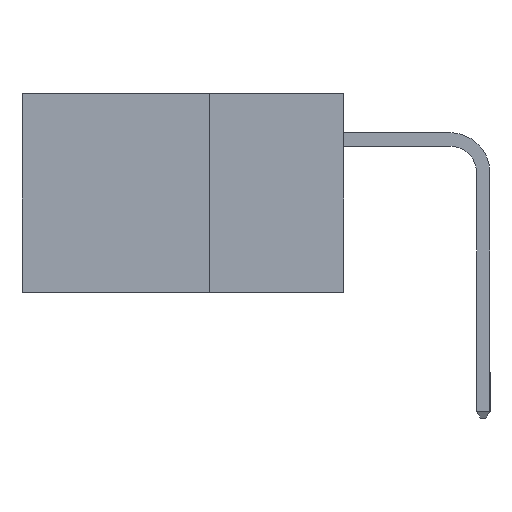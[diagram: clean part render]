
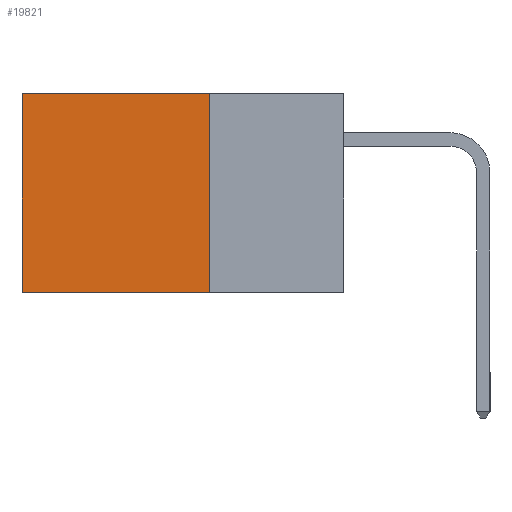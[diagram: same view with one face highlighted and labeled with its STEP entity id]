
A CAD part, left-side view. The second image highlights one B-rep face of the part: STEP entity #19821.
In plain terms, the highlighted planar face has unit normal (-1, 0, 0).
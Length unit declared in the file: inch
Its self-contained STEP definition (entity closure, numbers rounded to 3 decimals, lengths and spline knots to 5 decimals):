
#83 = CARTESIAN_POINT ( 'NONE',  ( 0.2615, 0.6, 0. ) ) ;
#1588 = DIRECTION ( 'NONE',  ( 0., 1., 0. ) ) ;
#1811 = DIRECTION ( 'NONE',  ( 0., 0., -1. ) ) ;
#2177 = VERTEX_POINT ( 'NONE', #6292 ) ;
#2209 = DIRECTION ( 'NONE',  ( 0., 1., 0. ) ) ;
#2489 = VECTOR ( 'NONE', #1811, 39.37008 ) ;
#2903 = ORIENTED_EDGE ( 'NONE', *, *, #11144, .F. ) ;
#2927 = CARTESIAN_POINT ( 'NONE',  ( 0.2615, 0.25, 0. ) ) ;
#2969 = PLANE ( 'NONE',  #20188 ) ;
#3796 = VECTOR ( 'NONE', #19532, 39.37008 ) ;
#4573 = CARTESIAN_POINT ( 'NONE',  ( 0.2615, 0.25, -0.37 ) ) ;
#5214 = LINE ( 'NONE', #22187, #18902 ) ;
#6292 = CARTESIAN_POINT ( 'NONE',  ( 0.2615, 0.25, -0.37 ) ) ;
#7425 = ORIENTED_EDGE ( 'NONE', *, *, #16064, .T. ) ;
#8316 = CARTESIAN_POINT ( 'NONE',  ( 0.2615, 0.25, -0.37 ) ) ;
#8417 = ORIENTED_EDGE ( 'NONE', *, *, #15539, .T. ) ;
#9429 = CARTESIAN_POINT ( 'NONE',  ( 0.2615, 0.6, -0.37 ) ) ;
#9544 = LINE ( 'NONE', #9429, #2489 ) ;
#9783 = VERTEX_POINT ( 'NONE', #83 ) ;
#11144 = EDGE_CURVE ( 'NONE', #11806, #2177, #15011, .T. ) ;
#11806 = VERTEX_POINT ( 'NONE', #2927 ) ;
#13011 = EDGE_CURVE ( 'NONE', #2177, #22037, #21641, .T. ) ;
#13561 = CARTESIAN_POINT ( 'NONE',  ( 0.2615, 0.6, -0.37 ) ) ;
#13758 = ORIENTED_EDGE ( 'NONE', *, *, #13011, .F. ) ;
#14237 = DIRECTION ( 'NONE',  ( 0., 0., -1. ) ) ;
#15011 = LINE ( 'NONE', #4573, #3796 ) ;
#15539 = EDGE_CURVE ( 'NONE', #11806, #9783, #5214, .T. ) ;
#16064 = EDGE_CURVE ( 'NONE', #9783, #22037, #9544, .T. ) ;
#18525 = EDGE_LOOP ( 'NONE', ( #7425, #13758, #2903, #8417 ) ) ;
#18902 = VECTOR ( 'NONE', #1588, 39.37008 ) ;
#19532 = DIRECTION ( 'NONE',  ( 0., 0., -1. ) ) ;
#19821 = ADVANCED_FACE ( 'NONE', ( #20166 ), #2969, .F. ) ;
#20166 = FACE_OUTER_BOUND ( 'NONE', #18525, .T. ) ;
#20188 = AXIS2_PLACEMENT_3D ( 'NONE', #24063, #21928, #14237 ) ;
#21641 = LINE ( 'NONE', #8316, #22842 ) ;
#21928 = DIRECTION ( 'NONE',  ( 1., 0., 0. ) ) ;
#22037 = VERTEX_POINT ( 'NONE', #13561 ) ;
#22187 = CARTESIAN_POINT ( 'NONE',  ( 0.2615, 0.25, 0. ) ) ;
#22842 = VECTOR ( 'NONE', #2209, 39.37008 ) ;
#24063 = CARTESIAN_POINT ( 'NONE',  ( 0.2615, 0.25, -0.37 ) ) ;
